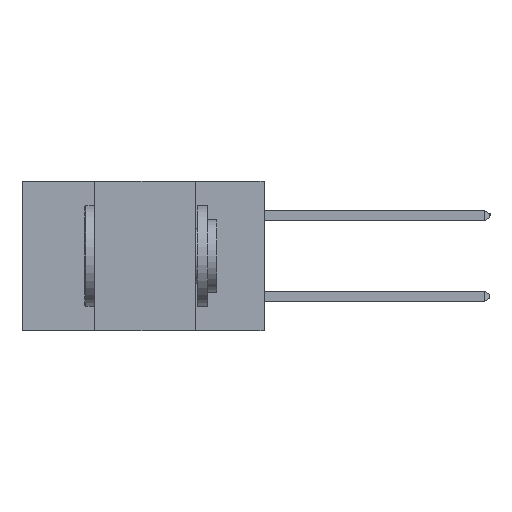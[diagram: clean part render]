
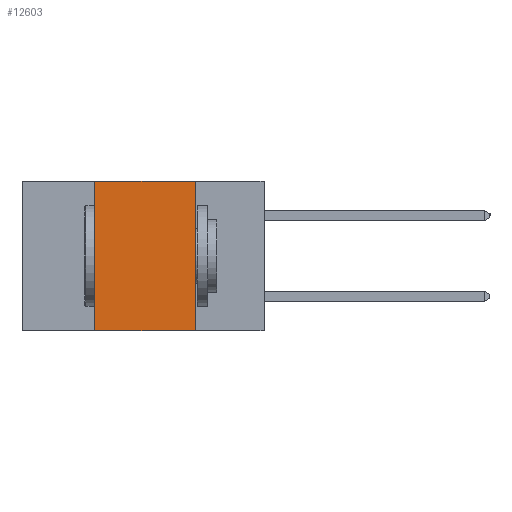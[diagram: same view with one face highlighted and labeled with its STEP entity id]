
A CAD part, left-side view. The second image highlights one B-rep face of the part: STEP entity #12603.
In plain terms, the highlighted planar face has unit normal (-1, 0, 0).
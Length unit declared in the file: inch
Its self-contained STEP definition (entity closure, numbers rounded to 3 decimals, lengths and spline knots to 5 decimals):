
#347 = VERTEX_POINT ( 'NONE', #14425 ) ;
#460 = CARTESIAN_POINT ( 'NONE',  ( 0., 0.42, -0.37 ) ) ;
#484 = ORIENTED_EDGE ( 'NONE', *, *, #10014, .F. ) ;
#584 = VECTOR ( 'NONE', #14613, 39.37008 ) ;
#888 = LINE ( 'NONE', #17387, #584 ) ;
#1179 = EDGE_CURVE ( 'NONE', #17129, #347, #7995, .T. ) ;
#1740 = LINE ( 'NONE', #10764, #18139 ) ;
#2019 = VERTEX_POINT ( 'NONE', #3168 ) ;
#2099 = DIRECTION ( 'NONE',  ( 1., 0., 0. ) ) ;
#2207 = ORIENTED_EDGE ( 'NONE', *, *, #1179, .F. ) ;
#2949 = CARTESIAN_POINT ( 'NONE',  ( 0., 0.6, 0. ) ) ;
#3168 = CARTESIAN_POINT ( 'NONE',  ( 0., 0.17, 0. ) ) ;
#3528 = AXIS2_PLACEMENT_3D ( 'NONE', #14319, #2099, #9446 ) ;
#3956 = EDGE_CURVE ( 'NONE', #17129, #8609, #1740, .T. ) ;
#6512 = DIRECTION ( 'NONE',  ( 0., 0., 1. ) ) ;
#7904 = VECTOR ( 'NONE', #6512, 39.37008 ) ;
#7995 = LINE ( 'NONE', #460, #7904 ) ;
#8590 = VECTOR ( 'NONE', #13500, 39.37008 ) ;
#8609 = VERTEX_POINT ( 'NONE', #17383 ) ;
#8808 = LINE ( 'NONE', #2949, #8590 ) ;
#9377 = DIRECTION ( 'NONE',  ( 0., -1., 0. ) ) ;
#9446 = DIRECTION ( 'NONE',  ( 0., 0., -1. ) ) ;
#9543 = CARTESIAN_POINT ( 'NONE',  ( 0., 0.42, -0.37 ) ) ;
#10014 = EDGE_CURVE ( 'NONE', #2019, #8609, #888, .T. ) ;
#10764 = CARTESIAN_POINT ( 'NONE',  ( 0., 0.6, -0.37 ) ) ;
#11042 = FACE_OUTER_BOUND ( 'NONE', #18998, .T. ) ;
#12039 = EDGE_CURVE ( 'NONE', #347, #2019, #8808, .T. ) ;
#12603 = ADVANCED_FACE ( 'NONE', ( #11042 ), #18603, .F. ) ;
#13500 = DIRECTION ( 'NONE',  ( 0., -1., 0. ) ) ;
#14319 = CARTESIAN_POINT ( 'NONE',  ( 0., 0.6, 0. ) ) ;
#14425 = CARTESIAN_POINT ( 'NONE',  ( 0., 0.42, 0. ) ) ;
#14613 = DIRECTION ( 'NONE',  ( 0., 0., -1. ) ) ;
#17129 = VERTEX_POINT ( 'NONE', #9543 ) ;
#17383 = CARTESIAN_POINT ( 'NONE',  ( 0., 0.17, -0.37 ) ) ;
#17387 = CARTESIAN_POINT ( 'NONE',  ( 0., 0.17, -0.37 ) ) ;
#18139 = VECTOR ( 'NONE', #9377, 39.37008 ) ;
#18455 = ORIENTED_EDGE ( 'NONE', *, *, #3956, .T. ) ;
#18603 = PLANE ( 'NONE',  #3528 ) ;
#18998 = EDGE_LOOP ( 'NONE', ( #484, #19207, #2207, #18455 ) ) ;
#19207 = ORIENTED_EDGE ( 'NONE', *, *, #12039, .F. ) ;
